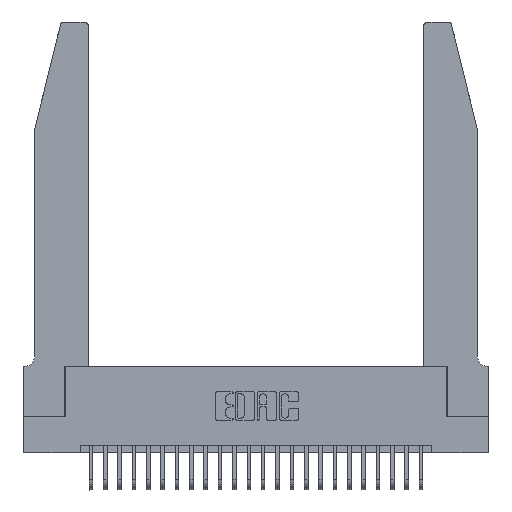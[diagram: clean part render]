
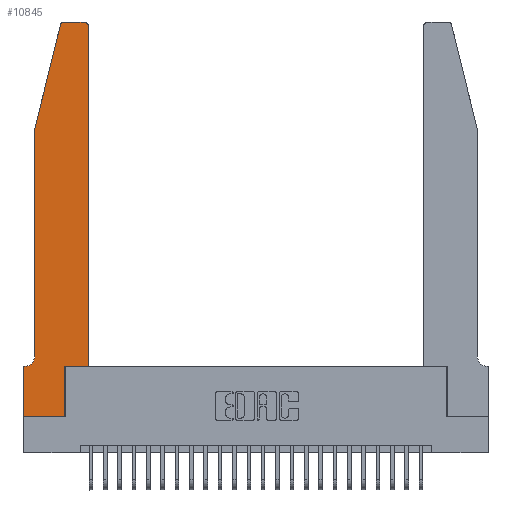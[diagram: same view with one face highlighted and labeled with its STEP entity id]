
A CAD part, top view. The second image highlights one B-rep face of the part: STEP entity #10845.
In plain terms, the highlighted planar face has unit normal (0, 0, 1).
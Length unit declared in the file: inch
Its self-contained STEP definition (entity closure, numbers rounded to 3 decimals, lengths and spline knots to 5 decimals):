
#112 = LINE ( 'NONE', #12942, #20962 ) ;
#329 = VERTEX_POINT ( 'NONE', #12048 ) ;
#640 = ORIENTED_EDGE ( 'NONE', *, *, #6362, .T. ) ;
#737 = EDGE_LOOP ( 'NONE', ( #23301, #3885, #12170, #20147, #22310, #13910, #640, #4292, #8524, #7473, #17269, #21761 ) ) ;
#741 = VECTOR ( 'NONE', #12344, 39.37008 ) ;
#819 = DIRECTION ( 'NONE',  ( 0., 0., 1. ) ) ;
#985 = LINE ( 'NONE', #15713, #21191 ) ;
#1753 = VERTEX_POINT ( 'NONE', #4764 ) ;
#1865 = VERTEX_POINT ( 'NONE', #24486 ) ;
#2365 = FACE_OUTER_BOUND ( 'NONE', #737, .T. ) ;
#2863 = AXIS2_PLACEMENT_3D ( 'NONE', #20571, #22510, #10894 ) ;
#3025 = AXIS2_PLACEMENT_3D ( 'NONE', #22974, #11363, #24921 ) ;
#3357 = VERTEX_POINT ( 'NONE', #23587 ) ;
#3364 = VERTEX_POINT ( 'NONE', #4085 ) ;
#3819 = CARTESIAN_POINT ( 'NONE',  ( 0., 0.35, 0.37 ) ) ;
#3885 = ORIENTED_EDGE ( 'NONE', *, *, #9897, .T. ) ;
#4085 = CARTESIAN_POINT ( 'NONE',  ( 0.4505, 0.35, 0.37 ) ) ;
#4292 = ORIENTED_EDGE ( 'NONE', *, *, #6985, .T. ) ;
#4764 = CARTESIAN_POINT ( 'NONE',  ( 0.0055, 0.35, 0.37 ) ) ;
#4792 = DIRECTION ( 'NONE',  ( 0., 0., -1. ) ) ;
#5150 = DIRECTION ( 'NONE',  ( -1., 0., 0. ) ) ;
#5310 = CARTESIAN_POINT ( 'NONE',  ( 0.4205, 2.75, 0.37 ) ) ;
#5859 = VERTEX_POINT ( 'NONE', #12175 ) ;
#6025 = LINE ( 'NONE', #14217, #741 ) ;
#6270 = CARTESIAN_POINT ( 'NONE',  ( 0.0755, 2., 0.37 ) ) ;
#6362 = EDGE_CURVE ( 'NONE', #19440, #3357, #985, .T. ) ;
#6917 = VERTEX_POINT ( 'NONE', #7481 ) ;
#6948 = EDGE_CURVE ( 'NONE', #1865, #14284, #8976, .T. ) ;
#6985 = EDGE_CURVE ( 'NONE', #3357, #8129, #8381, .T. ) ;
#7473 = ORIENTED_EDGE ( 'NONE', *, *, #10278, .T. ) ;
#7481 = CARTESIAN_POINT ( 'NONE',  ( 0.25487, 2.72718, 0.37 ) ) ;
#7920 = DIRECTION ( 'NONE',  ( 0., -1., 0. ) ) ;
#8115 = VECTOR ( 'NONE', #23583, 39.37008 ) ;
#8129 = VERTEX_POINT ( 'NONE', #9543 ) ;
#8251 = DIRECTION ( 'NONE',  ( -0.239, -0.971, 0. ) ) ;
#8381 = LINE ( 'NONE', #25207, #18155 ) ;
#8497 = EDGE_CURVE ( 'NONE', #5859, #18862, #14776, .T. ) ;
#8502 = CARTESIAN_POINT ( 'NONE',  ( 0.2865, 0.35, 0.37 ) ) ;
#8524 = ORIENTED_EDGE ( 'NONE', *, *, #11589, .T. ) ;
#8936 = VERTEX_POINT ( 'NONE', #8502 ) ;
#8976 = LINE ( 'NONE', #23194, #23882 ) ;
#9543 = CARTESIAN_POINT ( 'NONE',  ( 0.2865, 0., 0.37 ) ) ;
#9602 = AXIS2_PLACEMENT_3D ( 'NONE', #16516, #4792, #18454 ) ;
#9897 = EDGE_CURVE ( 'NONE', #329, #6917, #23775, .T. ) ;
#10067 = VECTOR ( 'NONE', #11002, 39.37008 ) ;
#10278 = EDGE_CURVE ( 'NONE', #8936, #3364, #20430, .T. ) ;
#10592 = EDGE_CURVE ( 'NONE', #6917, #1865, #13126, .T. ) ;
#10845 = ADVANCED_FACE ( 'NONE', ( #2365 ), #18647, .T. ) ;
#10894 = DIRECTION ( 'NONE',  ( 1., 0., 0. ) ) ;
#11002 = DIRECTION ( 'NONE',  ( 1., 0., 0. ) ) ;
#11363 = DIRECTION ( 'NONE',  ( 0., 0., 1. ) ) ;
#11589 = EDGE_CURVE ( 'NONE', #8129, #8936, #6025, .T. ) ;
#12048 = CARTESIAN_POINT ( 'NONE',  ( 0.284, 2.75, 0.37 ) ) ;
#12170 = ORIENTED_EDGE ( 'NONE', *, *, #10592, .T. ) ;
#12175 = CARTESIAN_POINT ( 'NONE',  ( 0.4505, 2.72, 0.37 ) ) ;
#12344 = DIRECTION ( 'NONE',  ( 0., 1., 0. ) ) ;
#12631 = CARTESIAN_POINT ( 'NONE',  ( 0.4205, 2.72, 0.37 ) ) ;
#12942 = CARTESIAN_POINT ( 'NONE',  ( 0.2605, 2.75, 0.37 ) ) ;
#13126 = LINE ( 'NONE', #6270, #22814 ) ;
#13910 = ORIENTED_EDGE ( 'NONE', *, *, #22784, .T. ) ;
#14217 = CARTESIAN_POINT ( 'NONE',  ( 0.2865, 0.35, 0.37 ) ) ;
#14284 = VERTEX_POINT ( 'NONE', #22752 ) ;
#14611 = CIRCLE ( 'NONE', #9602, 0.07 ) ;
#14612 = DIRECTION ( 'NONE',  ( 1., 0., 0. ) ) ;
#14653 = DIRECTION ( 'NONE',  ( -1., 0., 0. ) ) ;
#14776 = CIRCLE ( 'NONE', #25040, 0.03 ) ;
#15713 = CARTESIAN_POINT ( 'NONE',  ( 0., 0., 0.37 ) ) ;
#16516 = CARTESIAN_POINT ( 'NONE',  ( 0.0055, 0.42, 0.37 ) ) ;
#17269 = ORIENTED_EDGE ( 'NONE', *, *, #20806, .T. ) ;
#18155 = VECTOR ( 'NONE', #19426, 39.37008 ) ;
#18454 = DIRECTION ( 'NONE',  ( -1., 0., 0. ) ) ;
#18647 = PLANE ( 'NONE',  #2863 ) ;
#18780 = EDGE_CURVE ( 'NONE', #18862, #329, #112, .T. ) ;
#18862 = VERTEX_POINT ( 'NONE', #5310 ) ;
#19257 = EDGE_CURVE ( 'NONE', #14284, #1753, #14611, .T. ) ;
#19426 = DIRECTION ( 'NONE',  ( 1., 0., 0. ) ) ;
#19440 = VERTEX_POINT ( 'NONE', #3819 ) ;
#19937 = LINE ( 'NONE', #22324, #24443 ) ;
#20147 = ORIENTED_EDGE ( 'NONE', *, *, #6948, .T. ) ;
#20430 = LINE ( 'NONE', #24558, #10067 ) ;
#20571 = CARTESIAN_POINT ( 'NONE',  ( 0., 0.35, 0.37 ) ) ;
#20806 = EDGE_CURVE ( 'NONE', #3364, #5859, #23013, .T. ) ;
#20962 = VECTOR ( 'NONE', #5150, 39.37008 ) ;
#21191 = VECTOR ( 'NONE', #7920, 39.37008 ) ;
#21637 = CARTESIAN_POINT ( 'NONE',  ( 0.4505, 0.35, 0.37 ) ) ;
#21761 = ORIENTED_EDGE ( 'NONE', *, *, #8497, .T. ) ;
#22310 = ORIENTED_EDGE ( 'NONE', *, *, #19257, .T. ) ;
#22324 = CARTESIAN_POINT ( 'NONE',  ( 0.0755, 0.35, 0.37 ) ) ;
#22510 = DIRECTION ( 'NONE',  ( 0., 0., 1. ) ) ;
#22752 = CARTESIAN_POINT ( 'NONE',  ( 0.0755, 0.42, 0.37 ) ) ;
#22784 = EDGE_CURVE ( 'NONE', #1753, #19440, #19937, .T. ) ;
#22814 = VECTOR ( 'NONE', #8251, 39.37008 ) ;
#22974 = CARTESIAN_POINT ( 'NONE',  ( 0.284, 2.72, 0.37 ) ) ;
#23013 = LINE ( 'NONE', #21637, #8115 ) ;
#23194 = CARTESIAN_POINT ( 'NONE',  ( 0.0755, 2., 0.37 ) ) ;
#23301 = ORIENTED_EDGE ( 'NONE', *, *, #18780, .T. ) ;
#23583 = DIRECTION ( 'NONE',  ( 0., 1., 0. ) ) ;
#23587 = CARTESIAN_POINT ( 'NONE',  ( 0., 0., 0.37 ) ) ;
#23775 = CIRCLE ( 'NONE', #3025, 0.03 ) ;
#23882 = VECTOR ( 'NONE', #25130, 39.37008 ) ;
#24443 = VECTOR ( 'NONE', #14653, 39.37008 ) ;
#24486 = CARTESIAN_POINT ( 'NONE',  ( 0.0755, 2., 0.37 ) ) ;
#24558 = CARTESIAN_POINT ( 'NONE',  ( 0.4505, 0.35, 0.37 ) ) ;
#24921 = DIRECTION ( 'NONE',  ( 1., 0., 0. ) ) ;
#25040 = AXIS2_PLACEMENT_3D ( 'NONE', #12631, #819, #14612 ) ;
#25130 = DIRECTION ( 'NONE',  ( 0., -1., 0. ) ) ;
#25207 = CARTESIAN_POINT ( 'NONE',  ( 0., 0., 0.37 ) ) ;
